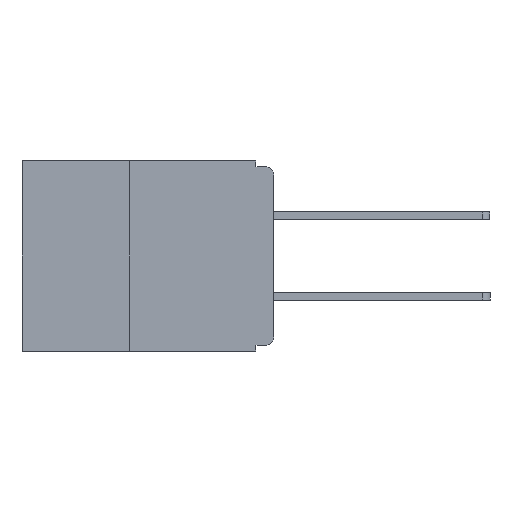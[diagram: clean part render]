
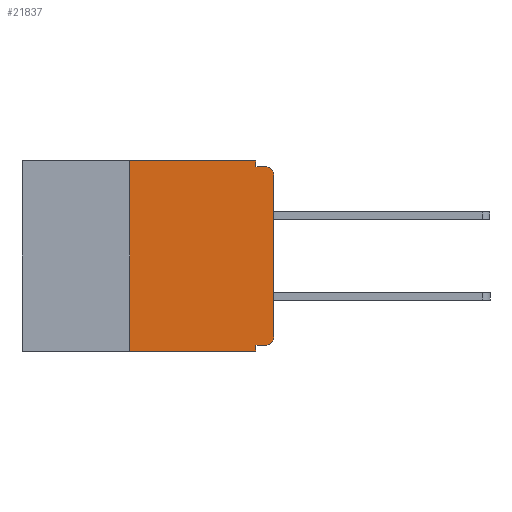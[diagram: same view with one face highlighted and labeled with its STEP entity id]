
A CAD part, left-side view. The second image highlights one B-rep face of the part: STEP entity #21837.
In plain terms, the highlighted planar face has unit normal (-1, 0, 0).
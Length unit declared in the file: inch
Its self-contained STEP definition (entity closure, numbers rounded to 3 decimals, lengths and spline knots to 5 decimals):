
#159 = CARTESIAN_POINT ( 'NONE',  ( 0., 0.25, 0. ) ) ;
#176 = LINE ( 'NONE', #12921, #24165 ) ;
#192 = ORIENTED_EDGE ( 'NONE', *, *, #11113, .T. ) ;
#438 = CARTESIAN_POINT ( 'NONE',  ( 0., 0.031, -0.33 ) ) ;
#656 = VERTEX_POINT ( 'NONE', #7603 ) ;
#688 = EDGE_CURVE ( 'NONE', #656, #21281, #16914, .T. ) ;
#1000 = CARTESIAN_POINT ( 'NONE',  ( 0., 0., -0.01 ) ) ;
#1310 = CARTESIAN_POINT ( 'NONE',  ( 0., 0.015, -0.305 ) ) ;
#1410 = CARTESIAN_POINT ( 'NONE',  ( 0., 0.031, 0. ) ) ;
#1840 = AXIS2_PLACEMENT_3D ( 'NONE', #24595, #22862, #11475 ) ;
#1951 = LINE ( 'NONE', #1000, #2588 ) ;
#2049 = LINE ( 'NONE', #13613, #22113 ) ;
#2588 = VECTOR ( 'NONE', #12872, 39.37008 ) ;
#3430 = ORIENTED_EDGE ( 'NONE', *, *, #19404, .F. ) ;
#3460 = CARTESIAN_POINT ( 'NONE',  ( 0., 0., -0.025 ) ) ;
#3476 = ORIENTED_EDGE ( 'NONE', *, *, #6335, .F. ) ;
#4183 = DIRECTION ( 'NONE',  ( -1., 0., 0. ) ) ;
#4186 = ORIENTED_EDGE ( 'NONE', *, *, #20616, .F. ) ;
#5008 = ORIENTED_EDGE ( 'NONE', *, *, #13434, .F. ) ;
#5068 = DIRECTION ( 'NONE',  ( 0., -1., 0. ) ) ;
#5479 = PLANE ( 'NONE',  #1840 ) ;
#5490 = DIRECTION ( 'NONE',  ( -1., 0., 0. ) ) ;
#5645 = DIRECTION ( 'NONE',  ( 0., 1., 0. ) ) ;
#5966 = VECTOR ( 'NONE', #8423, 39.37008 ) ;
#6208 = AXIS2_PLACEMENT_3D ( 'NONE', #1310, #5490, #18785 ) ;
#6335 = EDGE_CURVE ( 'NONE', #17701, #24247, #6605, .T. ) ;
#6440 = CARTESIAN_POINT ( 'NONE',  ( 0., 0.031, 0. ) ) ;
#6605 = LINE ( 'NONE', #6440, #5966 ) ;
#6744 = DIRECTION ( 'NONE',  ( 0., 0., 1. ) ) ;
#6984 = VERTEX_POINT ( 'NONE', #12298 ) ;
#7201 = ORIENTED_EDGE ( 'NONE', *, *, #14435, .T. ) ;
#7539 = ORIENTED_EDGE ( 'NONE', *, *, #24767, .F. ) ;
#7603 = CARTESIAN_POINT ( 'NONE',  ( 0., 0.015, -0.32 ) ) ;
#7790 = DIRECTION ( 'NONE',  ( 0., 0., 1. ) ) ;
#7805 = CIRCLE ( 'NONE', #10991, 0.015 ) ;
#7893 = ORIENTED_EDGE ( 'NONE', *, *, #8014, .F. ) ;
#8014 = EDGE_CURVE ( 'NONE', #656, #24730, #23061, .T. ) ;
#8423 = DIRECTION ( 'NONE',  ( 0., 0., -1. ) ) ;
#8932 = ORIENTED_EDGE ( 'NONE', *, *, #688, .T. ) ;
#9068 = VECTOR ( 'NONE', #15277, 39.37008 ) ;
#9467 = CARTESIAN_POINT ( 'NONE',  ( 0., 0.437, 0. ) ) ;
#9687 = VERTEX_POINT ( 'NONE', #159 ) ;
#9824 = EDGE_LOOP ( 'NONE', ( #22735, #192, #3430, #3476, #4186, #5008, #7201, #7539, #7893, #8932 ) ) ;
#10991 = AXIS2_PLACEMENT_3D ( 'NONE', #15873, #4183, #17746 ) ;
#11113 = EDGE_CURVE ( 'NONE', #15168, #19615, #7805, .T. ) ;
#11475 = DIRECTION ( 'NONE',  ( 0., 0., -1. ) ) ;
#11560 = CARTESIAN_POINT ( 'NONE',  ( 0., 0., -0.32 ) ) ;
#11590 = CARTESIAN_POINT ( 'NONE',  ( 0., 0., -0.305 ) ) ;
#12298 = CARTESIAN_POINT ( 'NONE',  ( 0., 0.031, -0.33 ) ) ;
#12872 = DIRECTION ( 'NONE',  ( 0., -1., 0. ) ) ;
#12921 = CARTESIAN_POINT ( 'NONE',  ( 0., 0.437, -0.33 ) ) ;
#13434 = EDGE_CURVE ( 'NONE', #17570, #9687, #2049, .T. ) ;
#13613 = CARTESIAN_POINT ( 'NONE',  ( 0., 0.25, -0.33 ) ) ;
#14435 = EDGE_CURVE ( 'NONE', #17570, #6984, #176, .T. ) ;
#14699 = CARTESIAN_POINT ( 'NONE',  ( 0., 0.25, -0.33 ) ) ;
#15168 = VERTEX_POINT ( 'NONE', #3460 ) ;
#15277 = DIRECTION ( 'NONE',  ( 0., -1., 0. ) ) ;
#15416 = LINE ( 'NONE', #9467, #9068 ) ;
#15873 = CARTESIAN_POINT ( 'NONE',  ( 0., 0.015, -0.025 ) ) ;
#15972 = CARTESIAN_POINT ( 'NONE',  ( 0., 0.031, -0.32 ) ) ;
#16052 = DIRECTION ( 'NONE',  ( 0., 0., -1. ) ) ;
#16914 = CIRCLE ( 'NONE', #6208, 0.015 ) ;
#17570 = VERTEX_POINT ( 'NONE', #14699 ) ;
#17701 = VERTEX_POINT ( 'NONE', #1410 ) ;
#17746 = DIRECTION ( 'NONE',  ( 0., 0., -1. ) ) ;
#17984 = VECTOR ( 'NONE', #5645, 39.37008 ) ;
#18013 = EDGE_CURVE ( 'NONE', #21281, #15168, #23874, .T. ) ;
#18036 = VECTOR ( 'NONE', #16052, 39.37008 ) ;
#18280 = CARTESIAN_POINT ( 'NONE',  ( 0., 0., 0. ) ) ;
#18785 = DIRECTION ( 'NONE',  ( 0., 0., -1. ) ) ;
#18806 = VECTOR ( 'NONE', #6744, 39.37008 ) ;
#19404 = EDGE_CURVE ( 'NONE', #24247, #19615, #1951, .T. ) ;
#19615 = VERTEX_POINT ( 'NONE', #21146 ) ;
#20305 = CARTESIAN_POINT ( 'NONE',  ( 0., 0.031, -0.01 ) ) ;
#20616 = EDGE_CURVE ( 'NONE', #9687, #17701, #15416, .T. ) ;
#21146 = CARTESIAN_POINT ( 'NONE',  ( 0., 0.015, -0.01 ) ) ;
#21155 = FACE_OUTER_BOUND ( 'NONE', #9824, .T. ) ;
#21281 = VERTEX_POINT ( 'NONE', #11590 ) ;
#21837 = ADVANCED_FACE ( 'NONE', ( #21155 ), #5479, .F. ) ;
#22113 = VECTOR ( 'NONE', #7790, 39.37008 ) ;
#22735 = ORIENTED_EDGE ( 'NONE', *, *, #18013, .T. ) ;
#22862 = DIRECTION ( 'NONE',  ( 1., 0., 0. ) ) ;
#23061 = LINE ( 'NONE', #11560, #17984 ) ;
#23386 = LINE ( 'NONE', #438, #18036 ) ;
#23874 = LINE ( 'NONE', #18280, #18806 ) ;
#24165 = VECTOR ( 'NONE', #5068, 39.37008 ) ;
#24247 = VERTEX_POINT ( 'NONE', #20305 ) ;
#24595 = CARTESIAN_POINT ( 'NONE',  ( 0., 0.437, 0. ) ) ;
#24730 = VERTEX_POINT ( 'NONE', #15972 ) ;
#24767 = EDGE_CURVE ( 'NONE', #24730, #6984, #23386, .T. ) ;
